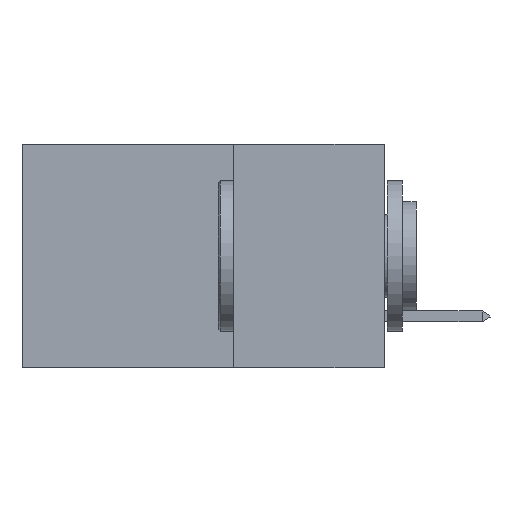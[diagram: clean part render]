
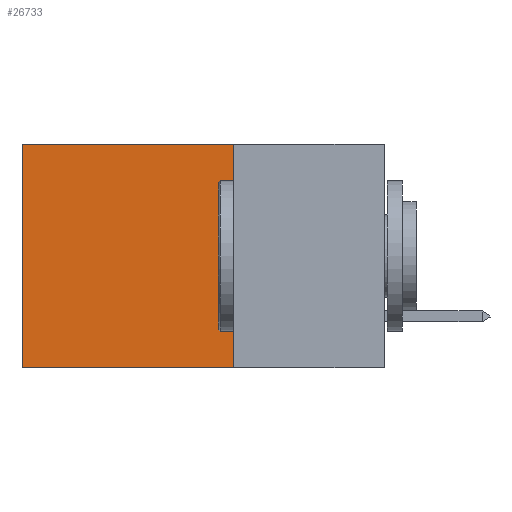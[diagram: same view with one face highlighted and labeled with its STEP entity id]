
A CAD part, left-side view. The second image highlights one B-rep face of the part: STEP entity #26733.
In plain terms, the highlighted planar face has unit normal (-1, 0, 0).
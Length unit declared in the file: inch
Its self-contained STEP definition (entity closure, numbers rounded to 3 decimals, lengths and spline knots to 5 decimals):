
#2218 = CARTESIAN_POINT ( 'NONE',  ( 0.2875, 0.25, -0.37 ) ) ;
#3105 = EDGE_CURVE ( 'NONE', #22501, #17598, #32877, .T. ) ;
#3416 = ORIENTED_EDGE ( 'NONE', *, *, #14650, .F. ) ;
#3594 = AXIS2_PLACEMENT_3D ( 'NONE', #31577, #39105, #13681 ) ;
#3852 = CARTESIAN_POINT ( 'NONE',  ( 0.2875, 0.25, 0. ) ) ;
#6731 = VECTOR ( 'NONE', #25863, 39.37008 ) ;
#8637 = CARTESIAN_POINT ( 'NONE',  ( 0.2875, 0.6, -0.37 ) ) ;
#8812 = DIRECTION ( 'NONE',  ( 0., 0., -1. ) ) ;
#10109 = PLANE ( 'NONE',  #3594 ) ;
#11751 = CARTESIAN_POINT ( 'NONE',  ( 0.2875, 0.25, 0. ) ) ;
#13681 = DIRECTION ( 'NONE',  ( 0., 0., -1. ) ) ;
#14650 = EDGE_CURVE ( 'NONE', #38836, #31646, #36177, .T. ) ;
#16787 = DIRECTION ( 'NONE',  ( 0., 1., 0. ) ) ;
#17598 = VERTEX_POINT ( 'NONE', #8637 ) ;
#17715 = CARTESIAN_POINT ( 'NONE',  ( 0.2875, 0.25, -0.37 ) ) ;
#19507 = VECTOR ( 'NONE', #16787, 39.37008 ) ;
#20368 = ORIENTED_EDGE ( 'NONE', *, *, #28001, .F. ) ;
#22501 = VERTEX_POINT ( 'NONE', #42710 ) ;
#23236 = CARTESIAN_POINT ( 'NONE',  ( 0.2875, 0.25, 0. ) ) ;
#25863 = DIRECTION ( 'NONE',  ( 0., 0., -1. ) ) ;
#26733 = ADVANCED_FACE ( 'NONE', ( #32820 ), #10109, .F. ) ;
#26935 = DIRECTION ( 'NONE',  ( 0., 1., 0. ) ) ;
#28001 = EDGE_CURVE ( 'NONE', #31646, #17598, #32781, .T. ) ;
#29984 = EDGE_CURVE ( 'NONE', #38836, #22501, #33939, .T. ) ;
#31577 = CARTESIAN_POINT ( 'NONE',  ( 0.2875, 0.25, 0. ) ) ;
#31646 = VERTEX_POINT ( 'NONE', #17715 ) ;
#32781 = LINE ( 'NONE', #2218, #19507 ) ;
#32820 = FACE_OUTER_BOUND ( 'NONE', #45642, .T. ) ;
#32877 = LINE ( 'NONE', #40738, #44961 ) ;
#33939 = LINE ( 'NONE', #23236, #36820 ) ;
#35354 = ORIENTED_EDGE ( 'NONE', *, *, #29984, .T. ) ;
#36177 = LINE ( 'NONE', #3852, #6731 ) ;
#36820 = VECTOR ( 'NONE', #26935, 39.37008 ) ;
#38836 = VERTEX_POINT ( 'NONE', #11751 ) ;
#39105 = DIRECTION ( 'NONE',  ( 1., 0., 0. ) ) ;
#40738 = CARTESIAN_POINT ( 'NONE',  ( 0.2875, 0.6, 0. ) ) ;
#42710 = CARTESIAN_POINT ( 'NONE',  ( 0.2875, 0.6, 0. ) ) ;
#44280 = ORIENTED_EDGE ( 'NONE', *, *, #3105, .T. ) ;
#44961 = VECTOR ( 'NONE', #8812, 39.37008 ) ;
#45642 = EDGE_LOOP ( 'NONE', ( #44280, #20368, #3416, #35354 ) ) ;
